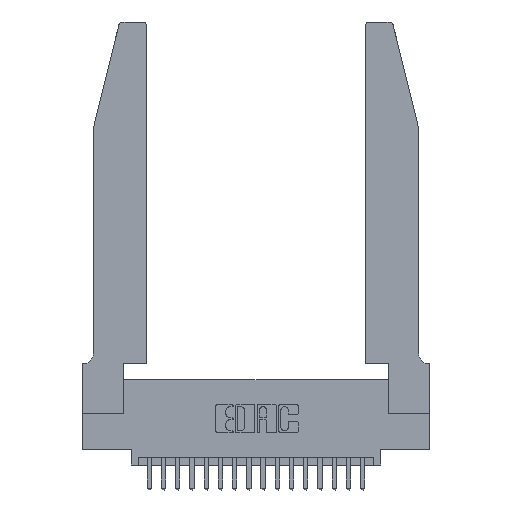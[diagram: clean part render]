
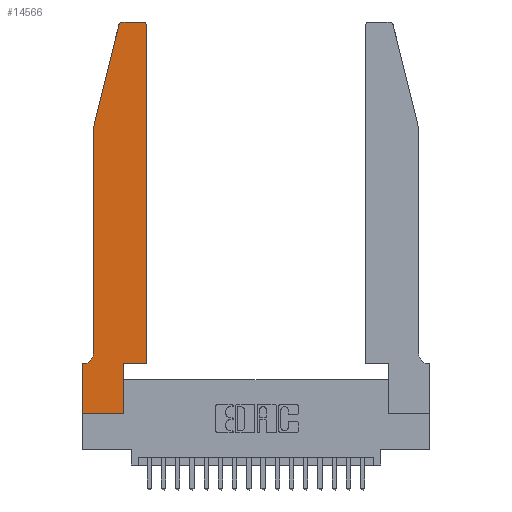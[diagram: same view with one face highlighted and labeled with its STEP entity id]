
A CAD part, top view. The second image highlights one B-rep face of the part: STEP entity #14566.
In plain terms, the highlighted planar face has unit normal (0, 0, 1).
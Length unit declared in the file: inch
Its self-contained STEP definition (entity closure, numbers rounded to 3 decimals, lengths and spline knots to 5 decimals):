
#129 = DIRECTION ( 'NONE',  ( 1., 0., 0. ) ) ;
#298 = DIRECTION ( 'NONE',  ( 0., 0., 1. ) ) ;
#427 = EDGE_CURVE ( 'NONE', #7359, #7843, #8693, .T. ) ;
#446 = CARTESIAN_POINT ( 'NONE',  ( 0.4505, 2.72, 0.37 ) ) ;
#671 = PLANE ( 'NONE',  #19462 ) ;
#728 = CARTESIAN_POINT ( 'NONE',  ( 0.2605, 2.75, 0.37 ) ) ;
#940 = ORIENTED_EDGE ( 'NONE', *, *, #3268, .T. ) ;
#1103 = CARTESIAN_POINT ( 'NONE',  ( 0.0755, 2., 0.37 ) ) ;
#1804 = ORIENTED_EDGE ( 'NONE', *, *, #2510, .T. ) ;
#1923 = CARTESIAN_POINT ( 'NONE',  ( 0.0755, 0.35, 0.37 ) ) ;
#2013 = AXIS2_PLACEMENT_3D ( 'NONE', #9030, #8507, #129 ) ;
#2038 = LINE ( 'NONE', #15720, #6375 ) ;
#2142 = DIRECTION ( 'NONE',  ( 0., 1., 0. ) ) ;
#2227 = CARTESIAN_POINT ( 'NONE',  ( 0.2865, 0., 0.37 ) ) ;
#2261 = ORIENTED_EDGE ( 'NONE', *, *, #9604, .T. ) ;
#2487 = CARTESIAN_POINT ( 'NONE',  ( 0.0055, 0.42, 0.37 ) ) ;
#2510 = EDGE_CURVE ( 'NONE', #15865, #19965, #2038, .T. ) ;
#2559 = CARTESIAN_POINT ( 'NONE',  ( 0.4505, 0.35, 0.37 ) ) ;
#3135 = EDGE_CURVE ( 'NONE', #14395, #20842, #20547, .T. ) ;
#3268 = EDGE_CURVE ( 'NONE', #15495, #5824, #15816, .T. ) ;
#3659 = VECTOR ( 'NONE', #5152, 39.37008 ) ;
#3897 = EDGE_CURVE ( 'NONE', #19965, #9379, #12053, .T. ) ;
#3997 = DIRECTION ( 'NONE',  ( 1., 0., 0. ) ) ;
#4150 = DIRECTION ( 'NONE',  ( -1., 0., 0. ) ) ;
#4325 = ORIENTED_EDGE ( 'NONE', *, *, #9265, .T. ) ;
#4397 = VECTOR ( 'NONE', #5698, 39.37008 ) ;
#4518 = EDGE_CURVE ( 'NONE', #9379, #7359, #7617, .T. ) ;
#4664 = ORIENTED_EDGE ( 'NONE', *, *, #427, .T. ) ;
#5152 = DIRECTION ( 'NONE',  ( 0., -1., 0. ) ) ;
#5210 = VERTEX_POINT ( 'NONE', #17061 ) ;
#5352 = CARTESIAN_POINT ( 'NONE',  ( 0., 0., 0.37 ) ) ;
#5698 = DIRECTION ( 'NONE',  ( 1., 0., 0. ) ) ;
#5824 = VERTEX_POINT ( 'NONE', #18648 ) ;
#5859 = ORIENTED_EDGE ( 'NONE', *, *, #3135, .T. ) ;
#6375 = VECTOR ( 'NONE', #6862, 39.37008 ) ;
#6418 = ORIENTED_EDGE ( 'NONE', *, *, #4518, .T. ) ;
#6862 = DIRECTION ( 'NONE',  ( 1., 0., 0. ) ) ;
#6959 = DIRECTION ( 'NONE',  ( 0., 1., 0. ) ) ;
#7203 = CARTESIAN_POINT ( 'NONE',  ( 0.0755, 2., 0.37 ) ) ;
#7276 = VECTOR ( 'NONE', #15491, 39.37008 ) ;
#7359 = VERTEX_POINT ( 'NONE', #2559 ) ;
#7617 = LINE ( 'NONE', #15489, #4397 ) ;
#7841 = ORIENTED_EDGE ( 'NONE', *, *, #11405, .T. ) ;
#7843 = VERTEX_POINT ( 'NONE', #446 ) ;
#7967 = EDGE_CURVE ( 'NONE', #19200, #15495, #11654, .T. ) ;
#8051 = LINE ( 'NONE', #1103, #16258 ) ;
#8507 = DIRECTION ( 'NONE',  ( 0., 0., 1. ) ) ;
#8693 = LINE ( 'NONE', #14211, #18403 ) ;
#9030 = CARTESIAN_POINT ( 'NONE',  ( 0.284, 2.72, 0.37 ) ) ;
#9255 = CIRCLE ( 'NONE', #16197, 0.07 ) ;
#9265 = EDGE_CURVE ( 'NONE', #5210, #14395, #9255, .T. ) ;
#9379 = VERTEX_POINT ( 'NONE', #14156 ) ;
#9604 = EDGE_CURVE ( 'NONE', #16154, #5210, #20398, .T. ) ;
#10104 = CARTESIAN_POINT ( 'NONE',  ( 0.4205, 2.72, 0.37 ) ) ;
#10270 = CARTESIAN_POINT ( 'NONE',  ( 0.2865, 0.35, 0.37 ) ) ;
#10412 = ORIENTED_EDGE ( 'NONE', *, *, #7967, .T. ) ;
#10973 = VECTOR ( 'NONE', #19959, 39.37008 ) ;
#11020 = VECTOR ( 'NONE', #2142, 39.37008 ) ;
#11405 = EDGE_CURVE ( 'NONE', #5824, #16154, #8051, .T. ) ;
#11554 = ORIENTED_EDGE ( 'NONE', *, *, #11705, .T. ) ;
#11654 = LINE ( 'NONE', #728, #7276 ) ;
#11705 = EDGE_CURVE ( 'NONE', #7843, #19200, #12157, .T. ) ;
#11768 = DIRECTION ( 'NONE',  ( 1., 0., 0. ) ) ;
#11991 = VECTOR ( 'NONE', #16285, 39.37008 ) ;
#12047 = ORIENTED_EDGE ( 'NONE', *, *, #3897, .T. ) ;
#12053 = LINE ( 'NONE', #10270, #11020 ) ;
#12128 = CARTESIAN_POINT ( 'NONE',  ( 0., 0.35, 0.37 ) ) ;
#12157 = CIRCLE ( 'NONE', #15548, 0.03 ) ;
#13753 = CARTESIAN_POINT ( 'NONE',  ( 0.284, 2.75, 0.37 ) ) ;
#13783 = DIRECTION ( 'NONE',  ( 0., 0., 1. ) ) ;
#13937 = DIRECTION ( 'NONE',  ( 0., 0., -1. ) ) ;
#14156 = CARTESIAN_POINT ( 'NONE',  ( 0.2865, 0.35, 0.37 ) ) ;
#14211 = CARTESIAN_POINT ( 'NONE',  ( 0.4505, 0.35, 0.37 ) ) ;
#14395 = VERTEX_POINT ( 'NONE', #14956 ) ;
#14566 = ADVANCED_FACE ( 'NONE', ( #18383 ), #671, .T. ) ;
#14615 = ORIENTED_EDGE ( 'NONE', *, *, #16735, .T. ) ;
#14722 = CARTESIAN_POINT ( 'NONE',  ( 0., 0.35, 0.37 ) ) ;
#14867 = EDGE_LOOP ( 'NONE', ( #10412, #940, #7841, #2261, #4325, #5859, #14615, #1804, #12047, #6418, #4664, #11554 ) ) ;
#14956 = CARTESIAN_POINT ( 'NONE',  ( 0.0055, 0.35, 0.37 ) ) ;
#15343 = LINE ( 'NONE', #5352, #10973 ) ;
#15489 = CARTESIAN_POINT ( 'NONE',  ( 0.4505, 0.35, 0.37 ) ) ;
#15491 = DIRECTION ( 'NONE',  ( -1., 0., 0. ) ) ;
#15495 = VERTEX_POINT ( 'NONE', #13753 ) ;
#15548 = AXIS2_PLACEMENT_3D ( 'NONE', #10104, #298, #11768 ) ;
#15720 = CARTESIAN_POINT ( 'NONE',  ( 0., 0., 0.37 ) ) ;
#15816 = CIRCLE ( 'NONE', #2013, 0.03 ) ;
#15865 = VERTEX_POINT ( 'NONE', #20738 ) ;
#16154 = VERTEX_POINT ( 'NONE', #7203 ) ;
#16197 = AXIS2_PLACEMENT_3D ( 'NONE', #2487, #13937, #4150 ) ;
#16258 = VECTOR ( 'NONE', #17244, 39.37008 ) ;
#16285 = DIRECTION ( 'NONE',  ( -1., 0., 0. ) ) ;
#16544 = CARTESIAN_POINT ( 'NONE',  ( 0.0755, 2., 0.37 ) ) ;
#16735 = EDGE_CURVE ( 'NONE', #20842, #15865, #15343, .T. ) ;
#17061 = CARTESIAN_POINT ( 'NONE',  ( 0.0755, 0.42, 0.37 ) ) ;
#17244 = DIRECTION ( 'NONE',  ( -0.239, -0.971, 0. ) ) ;
#18148 = CARTESIAN_POINT ( 'NONE',  ( 0.4205, 2.75, 0.37 ) ) ;
#18383 = FACE_OUTER_BOUND ( 'NONE', #14867, .T. ) ;
#18403 = VECTOR ( 'NONE', #6959, 39.37008 ) ;
#18648 = CARTESIAN_POINT ( 'NONE',  ( 0.25487, 2.72718, 0.37 ) ) ;
#19200 = VERTEX_POINT ( 'NONE', #18148 ) ;
#19462 = AXIS2_PLACEMENT_3D ( 'NONE', #12128, #13783, #3997 ) ;
#19959 = DIRECTION ( 'NONE',  ( 0., -1., 0. ) ) ;
#19965 = VERTEX_POINT ( 'NONE', #2227 ) ;
#20398 = LINE ( 'NONE', #16544, #3659 ) ;
#20547 = LINE ( 'NONE', #1923, #11991 ) ;
#20738 = CARTESIAN_POINT ( 'NONE',  ( 0., 0., 0.37 ) ) ;
#20842 = VERTEX_POINT ( 'NONE', #14722 ) ;
